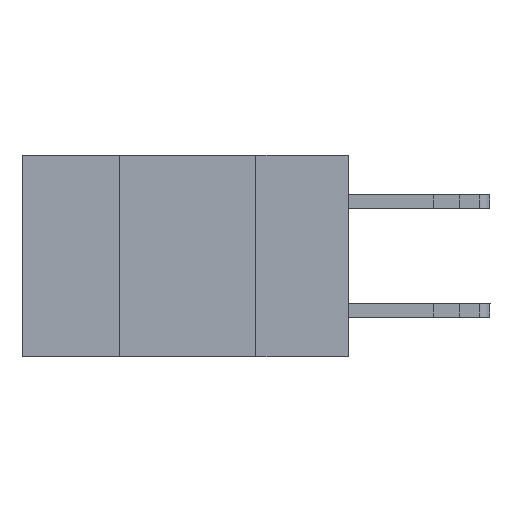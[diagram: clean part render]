
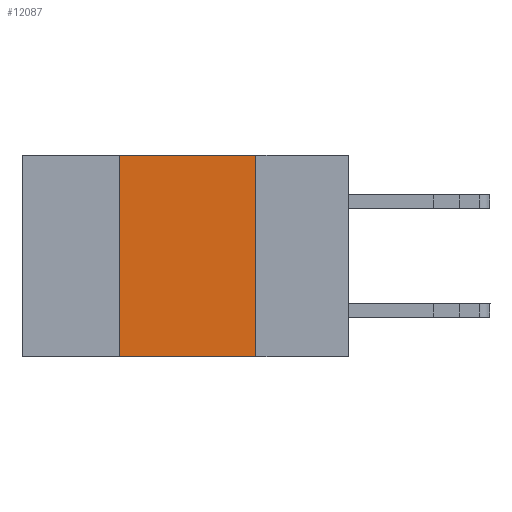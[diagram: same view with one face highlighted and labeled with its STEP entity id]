
A CAD part, left-side view. The second image highlights one B-rep face of the part: STEP entity #12087.
In plain terms, the highlighted planar face has unit normal (-1, 0, 0).
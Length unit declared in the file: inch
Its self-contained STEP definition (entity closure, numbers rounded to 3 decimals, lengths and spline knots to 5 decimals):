
#41 = EDGE_LOOP ( 'NONE', ( #4648, #2276, #4841, #11451 ) ) ;
#602 = VERTEX_POINT ( 'NONE', #2436 ) ;
#728 = EDGE_CURVE ( 'NONE', #602, #11231, #9394, .T. ) ;
#1218 = DIRECTION ( 'NONE',  ( 1., 0., 0. ) ) ;
#1273 = CARTESIAN_POINT ( 'NONE',  ( 0., 0.42, -0.37 ) ) ;
#1418 = AXIS2_PLACEMENT_3D ( 'NONE', #4262, #1218, #8401 ) ;
#1742 = EDGE_CURVE ( 'NONE', #11231, #3743, #12544, .T. ) ;
#2276 = ORIENTED_EDGE ( 'NONE', *, *, #728, .F. ) ;
#2436 = CARTESIAN_POINT ( 'NONE',  ( 0., 0.42, 0. ) ) ;
#2834 = CARTESIAN_POINT ( 'NONE',  ( 0., 0.17, -0.37 ) ) ;
#3027 = LINE ( 'NONE', #5898, #3674 ) ;
#3124 = DIRECTION ( 'NONE',  ( 0., 0., -1. ) ) ;
#3169 = LINE ( 'NONE', #8846, #6564 ) ;
#3547 = CARTESIAN_POINT ( 'NONE',  ( 0., 0.6, 0. ) ) ;
#3674 = VECTOR ( 'NONE', #6923, 39.37008 ) ;
#3743 = VERTEX_POINT ( 'NONE', #2834 ) ;
#4262 = CARTESIAN_POINT ( 'NONE',  ( 0., 0.6, 0. ) ) ;
#4648 = ORIENTED_EDGE ( 'NONE', *, *, #1742, .F. ) ;
#4841 = ORIENTED_EDGE ( 'NONE', *, *, #11934, .F. ) ;
#5898 = CARTESIAN_POINT ( 'NONE',  ( 0., 0.42, 0. ) ) ;
#6564 = VECTOR ( 'NONE', #9841, 39.37008 ) ;
#6923 = DIRECTION ( 'NONE',  ( 0., 0., 1. ) ) ;
#7583 = VECTOR ( 'NONE', #3124, 39.37008 ) ;
#7929 = VECTOR ( 'NONE', #12769, 39.37008 ) ;
#8401 = DIRECTION ( 'NONE',  ( 0., 0., -1. ) ) ;
#8846 = CARTESIAN_POINT ( 'NONE',  ( 0., 0.6, -0.37 ) ) ;
#9130 = VERTEX_POINT ( 'NONE', #1273 ) ;
#9394 = LINE ( 'NONE', #3547, #7929 ) ;
#9417 = PLANE ( 'NONE',  #1418 ) ;
#9841 = DIRECTION ( 'NONE',  ( 0., -1., 0. ) ) ;
#10425 = CARTESIAN_POINT ( 'NONE',  ( 0., 0.17, 0. ) ) ;
#10910 = FACE_OUTER_BOUND ( 'NONE', #41, .T. ) ;
#11057 = CARTESIAN_POINT ( 'NONE',  ( 0., 0.17, 0. ) ) ;
#11231 = VERTEX_POINT ( 'NONE', #11057 ) ;
#11451 = ORIENTED_EDGE ( 'NONE', *, *, #12585, .T. ) ;
#11934 = EDGE_CURVE ( 'NONE', #9130, #602, #3027, .T. ) ;
#12087 = ADVANCED_FACE ( 'NONE', ( #10910 ), #9417, .F. ) ;
#12544 = LINE ( 'NONE', #10425, #7583 ) ;
#12585 = EDGE_CURVE ( 'NONE', #9130, #3743, #3169, .T. ) ;
#12769 = DIRECTION ( 'NONE',  ( 0., -1., 0. ) ) ;
